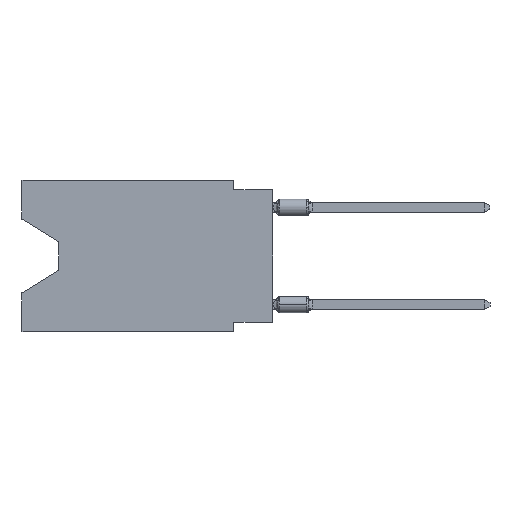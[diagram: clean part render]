
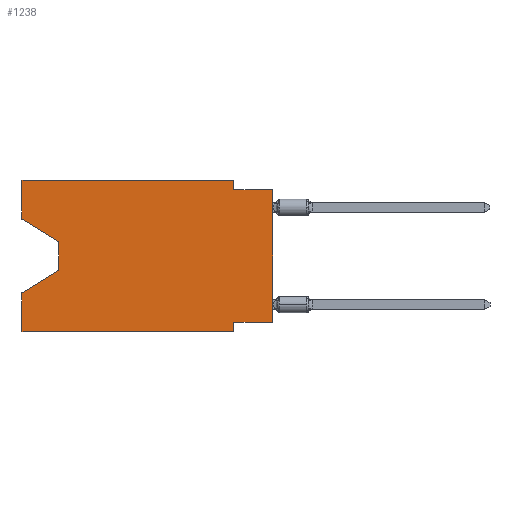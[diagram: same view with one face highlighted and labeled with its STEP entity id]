
A CAD part, left-side view. The second image highlights one B-rep face of the part: STEP entity #1238.
In plain terms, the highlighted planar face has unit normal (-1, 0, 0).
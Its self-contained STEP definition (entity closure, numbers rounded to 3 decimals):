
#39 = LINE ( 'NONE', #18742, #17565 ) ;
#260 = EDGE_CURVE ( 'NONE', #19238, #1253, #2261, .T. ) ;
#506 = AXIS2_PLACEMENT_3D ( 'NONE', #4302, #7142, #17852 ) ;
#540 = VECTOR ( 'NONE', #1563, 1000. ) ;
#644 = VERTEX_POINT ( 'NONE', #16160 ) ;
#852 = VECTOR ( 'NONE', #6390, 1000. ) ;
#1238 = ADVANCED_FACE ( 'NONE', ( #4111 ), #14818, .F. ) ;
#1253 = VERTEX_POINT ( 'NONE', #11057 ) ;
#1274 = LINE ( 'NONE', #9151, #11790 ) ;
#1403 = ORIENTED_EDGE ( 'NONE', *, *, #18633, .T. ) ;
#1543 = DIRECTION ( 'NONE',  ( 0., 0., 1. ) ) ;
#1563 = DIRECTION ( 'NONE',  ( 0., -0.855, -0.519 ) ) ;
#2124 = VERTEX_POINT ( 'NONE', #5055 ) ;
#2261 = LINE ( 'NONE', #6429, #16985 ) ;
#2439 = CARTESIAN_POINT ( 'NONE',  ( 0., 2.54, -9.271 ) ) ;
#2532 = LINE ( 'NONE', #19519, #15797 ) ;
#2680 = VECTOR ( 'NONE', #2845, 1000. ) ;
#2725 = VECTOR ( 'NONE', #7597, 1000. ) ;
#2845 = DIRECTION ( 'NONE',  ( 0., 0., -1. ) ) ;
#2975 = LINE ( 'NONE', #9232, #6533 ) ;
#3143 = DIRECTION ( 'NONE',  ( 0., -1., 0. ) ) ;
#4054 = LINE ( 'NONE', #8590, #17285 ) ;
#4111 = FACE_OUTER_BOUND ( 'NONE', #4435, .T. ) ;
#4256 = VERTEX_POINT ( 'NONE', #16868 ) ;
#4284 = VECTOR ( 'NONE', #3143, 1000. ) ;
#4302 = CARTESIAN_POINT ( 'NONE',  ( 0., 16.383, 0. ) ) ;
#4328 = CARTESIAN_POINT ( 'NONE',  ( 0., 16.383, -7.36 ) ) ;
#4435 = EDGE_LOOP ( 'NONE', ( #10798, #15714, #14133, #14865, #14843, #16675, #6878, #1403, #19867, #7293, #15367, #17861 ) ) ;
#4591 = DIRECTION ( 'NONE',  ( 0., -1., 0. ) ) ;
#5055 = CARTESIAN_POINT ( 'NONE',  ( 0., 13.97, -4.013 ) ) ;
#5298 = EDGE_CURVE ( 'NONE', #2124, #5917, #2532, .T. ) ;
#5671 = DIRECTION ( 'NONE',  ( 0., 0., -1. ) ) ;
#5824 = VERTEX_POINT ( 'NONE', #4328 ) ;
#5917 = VERTEX_POINT ( 'NONE', #14010 ) ;
#6236 = CARTESIAN_POINT ( 'NONE',  ( 0., 16.383, -2.546 ) ) ;
#6329 = VECTOR ( 'NONE', #17557, 1000. ) ;
#6390 = DIRECTION ( 'NONE',  ( 0., 1., 0. ) ) ;
#6429 = CARTESIAN_POINT ( 'NONE',  ( 0., 16.383, 0. ) ) ;
#6533 = VECTOR ( 'NONE', #1543, 1000. ) ;
#6878 = ORIENTED_EDGE ( 'NONE', *, *, #10333, .F. ) ;
#7142 = DIRECTION ( 'NONE',  ( 1., 0., 0. ) ) ;
#7246 = VERTEX_POINT ( 'NONE', #8508 ) ;
#7293 = ORIENTED_EDGE ( 'NONE', *, *, #14152, .F. ) ;
#7597 = DIRECTION ( 'NONE',  ( 0., 0.855, -0.519 ) ) ;
#8508 = CARTESIAN_POINT ( 'NONE',  ( 0., 0., -9.271 ) ) ;
#8590 = CARTESIAN_POINT ( 'NONE',  ( 0., 0., 0. ) ) ;
#8881 = DIRECTION ( 'NONE',  ( 0., 0., 1. ) ) ;
#9094 = LINE ( 'NONE', #15280, #2725 ) ;
#9112 = CARTESIAN_POINT ( 'NONE',  ( 0., 2.54, -9.906 ) ) ;
#9151 = CARTESIAN_POINT ( 'NONE',  ( 0., 16.383, -9.906 ) ) ;
#9232 = CARTESIAN_POINT ( 'NONE',  ( 0., 16.383, 0. ) ) ;
#10333 = EDGE_CURVE ( 'NONE', #7246, #19784, #12730, .T. ) ;
#10681 = EDGE_CURVE ( 'NONE', #19238, #2124, #14201, .T. ) ;
#10745 = CARTESIAN_POINT ( 'NONE',  ( 0., 0., -0.635 ) ) ;
#10798 = ORIENTED_EDGE ( 'NONE', *, *, #10681, .T. ) ;
#11023 = VERTEX_POINT ( 'NONE', #10745 ) ;
#11057 = CARTESIAN_POINT ( 'NONE',  ( 0., 16.383, 0. ) ) ;
#11480 = CARTESIAN_POINT ( 'NONE',  ( 0., 2.54, -9.906 ) ) ;
#11527 = EDGE_CURVE ( 'NONE', #5917, #5824, #9094, .T. ) ;
#11790 = VECTOR ( 'NONE', #15440, 1000. ) ;
#12223 = EDGE_CURVE ( 'NONE', #4256, #19622, #1274, .T. ) ;
#12433 = LINE ( 'NONE', #18606, #2680 ) ;
#12730 = LINE ( 'NONE', #18809, #852 ) ;
#14010 = CARTESIAN_POINT ( 'NONE',  ( 0., 13.97, -5.893 ) ) ;
#14133 = ORIENTED_EDGE ( 'NONE', *, *, #11527, .T. ) ;
#14152 = EDGE_CURVE ( 'NONE', #15556, #644, #12433, .T. ) ;
#14201 = LINE ( 'NONE', #6236, #540 ) ;
#14492 = DIRECTION ( 'NONE',  ( 0., 0., 1. ) ) ;
#14818 = PLANE ( 'NONE',  #506 ) ;
#14843 = ORIENTED_EDGE ( 'NONE', *, *, #12223, .T. ) ;
#14865 = ORIENTED_EDGE ( 'NONE', *, *, #15905, .F. ) ;
#15232 = EDGE_CURVE ( 'NONE', #1253, #15556, #16979, .T. ) ;
#15280 = CARTESIAN_POINT ( 'NONE',  ( 0., 13.97, -5.893 ) ) ;
#15367 = ORIENTED_EDGE ( 'NONE', *, *, #15232, .F. ) ;
#15374 = CARTESIAN_POINT ( 'NONE',  ( 0., 16.383, 0. ) ) ;
#15440 = DIRECTION ( 'NONE',  ( 0., -1., 0. ) ) ;
#15556 = VERTEX_POINT ( 'NONE', #18669 ) ;
#15714 = ORIENTED_EDGE ( 'NONE', *, *, #5298, .T. ) ;
#15797 = VECTOR ( 'NONE', #5671, 1000. ) ;
#15905 = EDGE_CURVE ( 'NONE', #4256, #5824, #2975, .T. ) ;
#16160 = CARTESIAN_POINT ( 'NONE',  ( 0., 2.54, -0.635 ) ) ;
#16675 = ORIENTED_EDGE ( 'NONE', *, *, #18909, .F. ) ;
#16868 = CARTESIAN_POINT ( 'NONE',  ( 0., 16.383, -9.906 ) ) ;
#16979 = LINE ( 'NONE', #15374, #4284 ) ;
#16985 = VECTOR ( 'NONE', #14492, 1000. ) ;
#17093 = EDGE_CURVE ( 'NONE', #644, #11023, #39, .T. ) ;
#17129 = CARTESIAN_POINT ( 'NONE',  ( 0., 16.383, -2.546 ) ) ;
#17285 = VECTOR ( 'NONE', #8881, 1000. ) ;
#17557 = DIRECTION ( 'NONE',  ( 0., 0., -1. ) ) ;
#17565 = VECTOR ( 'NONE', #4591, 1000. ) ;
#17852 = DIRECTION ( 'NONE',  ( 0., 0., -1. ) ) ;
#17861 = ORIENTED_EDGE ( 'NONE', *, *, #260, .F. ) ;
#18606 = CARTESIAN_POINT ( 'NONE',  ( 0., 2.54, 0. ) ) ;
#18633 = EDGE_CURVE ( 'NONE', #7246, #11023, #4054, .T. ) ;
#18669 = CARTESIAN_POINT ( 'NONE',  ( 0., 2.54, 0. ) ) ;
#18742 = CARTESIAN_POINT ( 'NONE',  ( 0., 0., -0.635 ) ) ;
#18809 = CARTESIAN_POINT ( 'NONE',  ( 0., 0., -9.271 ) ) ;
#18909 = EDGE_CURVE ( 'NONE', #19784, #19622, #19175, .T. ) ;
#19175 = LINE ( 'NONE', #11480, #6329 ) ;
#19238 = VERTEX_POINT ( 'NONE', #17129 ) ;
#19519 = CARTESIAN_POINT ( 'NONE',  ( 0., 13.97, -4.013 ) ) ;
#19622 = VERTEX_POINT ( 'NONE', #9112 ) ;
#19784 = VERTEX_POINT ( 'NONE', #2439 ) ;
#19867 = ORIENTED_EDGE ( 'NONE', *, *, #17093, .F. ) ;
